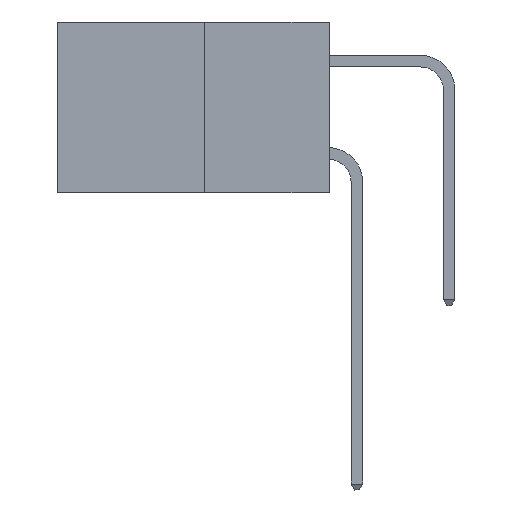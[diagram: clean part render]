
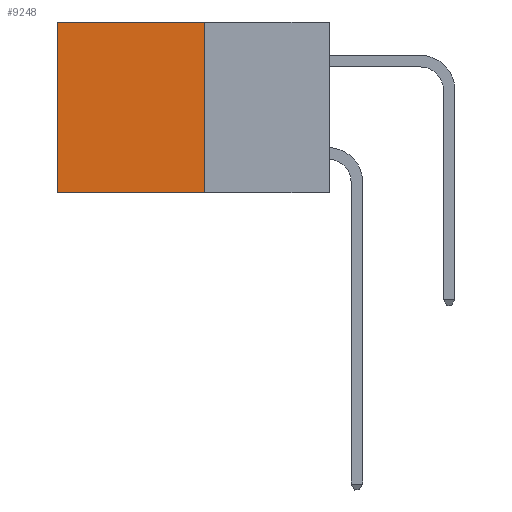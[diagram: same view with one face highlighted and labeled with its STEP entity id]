
A CAD part, left-side view. The second image highlights one B-rep face of the part: STEP entity #9248.
In plain terms, the highlighted planar face has unit normal (-1, 0, 0).
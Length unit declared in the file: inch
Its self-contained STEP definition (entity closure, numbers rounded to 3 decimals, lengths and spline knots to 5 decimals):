
#2 = PLANE ( 'NONE',  #8891 ) ;
#44 = DIRECTION ( 'NONE',  ( 0., 0., -1. ) ) ;
#179 = DIRECTION ( 'NONE',  ( 1., 0., 0. ) ) ;
#313 = CARTESIAN_POINT ( 'NONE',  ( 0.277, 0.27, -0.37 ) ) ;
#680 = EDGE_CURVE ( 'NONE', #7699, #791, #9183, .T. ) ;
#791 = VERTEX_POINT ( 'NONE', #4611 ) ;
#923 = CARTESIAN_POINT ( 'NONE',  ( 0.277, 0.27, -0.37 ) ) ;
#1128 = ORIENTED_EDGE ( 'NONE', *, *, #3179, .F. ) ;
#1160 = ORIENTED_EDGE ( 'NONE', *, *, #1837, .F. ) ;
#1837 = EDGE_CURVE ( 'NONE', #3780, #791, #2275, .T. ) ;
#1881 = CARTESIAN_POINT ( 'NONE',  ( 0.277, 0.27, 0. ) ) ;
#2161 = ORIENTED_EDGE ( 'NONE', *, *, #9129, .T. ) ;
#2257 = DIRECTION ( 'NONE',  ( 0., 0., -1. ) ) ;
#2275 = LINE ( 'NONE', #923, #4355 ) ;
#2320 = CARTESIAN_POINT ( 'NONE',  ( 0.277, 0.27, -0.37 ) ) ;
#2680 = EDGE_LOOP ( 'NONE', ( #5845, #1160, #1128, #2161 ) ) ;
#2752 = VERTEX_POINT ( 'NONE', #1881 ) ;
#3179 = EDGE_CURVE ( 'NONE', #2752, #3780, #9267, .T. ) ;
#3487 = DIRECTION ( 'NONE',  ( 0., 0., -1. ) ) ;
#3780 = VERTEX_POINT ( 'NONE', #8423 ) ;
#3890 = VECTOR ( 'NONE', #4148, 39.37008 ) ;
#4148 = DIRECTION ( 'NONE',  ( 0., 1., 0. ) ) ;
#4355 = VECTOR ( 'NONE', #5968, 39.37008 ) ;
#4611 = CARTESIAN_POINT ( 'NONE',  ( 0.277, 0.59, -0.37 ) ) ;
#5558 = VECTOR ( 'NONE', #3487, 39.37008 ) ;
#5845 = ORIENTED_EDGE ( 'NONE', *, *, #680, .T. ) ;
#5968 = DIRECTION ( 'NONE',  ( 0., 1., 0. ) ) ;
#7307 = VECTOR ( 'NONE', #2257, 39.37008 ) ;
#7422 = CARTESIAN_POINT ( 'NONE',  ( 0.277, 0.59, 0. ) ) ;
#7699 = VERTEX_POINT ( 'NONE', #7422 ) ;
#8137 = CARTESIAN_POINT ( 'NONE',  ( 0.277, 0.27, 0. ) ) ;
#8423 = CARTESIAN_POINT ( 'NONE',  ( 0.277, 0.27, -0.37 ) ) ;
#8891 = AXIS2_PLACEMENT_3D ( 'NONE', #313, #179, #44 ) ;
#9129 = EDGE_CURVE ( 'NONE', #2752, #7699, #9505, .T. ) ;
#9183 = LINE ( 'NONE', #9655, #5558 ) ;
#9248 = ADVANCED_FACE ( 'NONE', ( #9598 ), #2, .F. ) ;
#9267 = LINE ( 'NONE', #2320, #7307 ) ;
#9505 = LINE ( 'NONE', #8137, #3890 ) ;
#9598 = FACE_OUTER_BOUND ( 'NONE', #2680, .T. ) ;
#9655 = CARTESIAN_POINT ( 'NONE',  ( 0.277, 0.59, -0.37 ) ) ;
